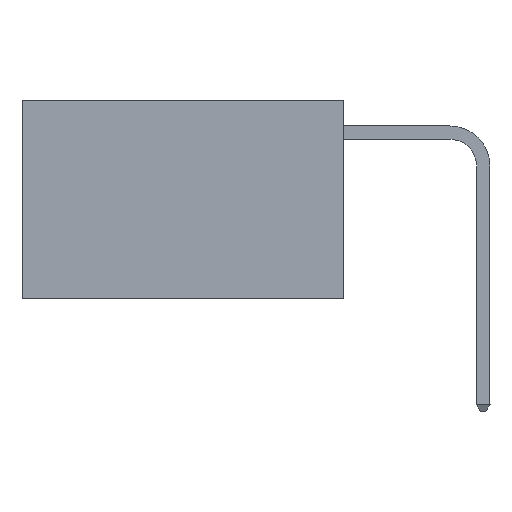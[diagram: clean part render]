
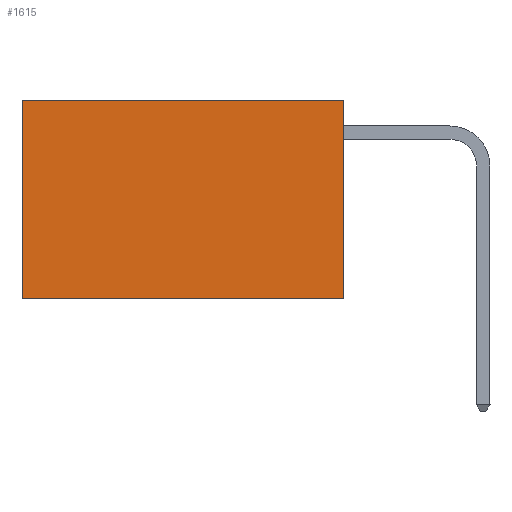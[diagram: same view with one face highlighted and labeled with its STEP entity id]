
A CAD part, left-side view. The second image highlights one B-rep face of the part: STEP entity #1615.
In plain terms, the highlighted planar face has unit normal (-1, 0, 0).
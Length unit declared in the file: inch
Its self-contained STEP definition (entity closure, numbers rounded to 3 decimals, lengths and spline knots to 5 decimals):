
#1 = LINE ( 'NONE', #4993, #1832 ) ;
#524 = CARTESIAN_POINT ( 'NONE',  ( 0.2625, 0., 0. ) ) ;
#731 = VERTEX_POINT ( 'NONE', #9139 ) ;
#1536 = CARTESIAN_POINT ( 'NONE',  ( 0.2625, 0.6, 0. ) ) ;
#1544 = VERTEX_POINT ( 'NONE', #2922 ) ;
#1615 = ADVANCED_FACE ( 'NONE', ( #4581 ), #5509, .F. ) ;
#1832 = VECTOR ( 'NONE', #2726, 39.37008 ) ;
#2323 = VECTOR ( 'NONE', #4527, 39.37008 ) ;
#2660 = DIRECTION ( 'NONE',  ( 1., 0., 0. ) ) ;
#2726 = DIRECTION ( 'NONE',  ( 0., 1., 0. ) ) ;
#2850 = VERTEX_POINT ( 'NONE', #5154 ) ;
#2922 = CARTESIAN_POINT ( 'NONE',  ( 0.2625, 0.6, 0. ) ) ;
#3022 = CARTESIAN_POINT ( 'NONE',  ( 0.2625, 0., 0. ) ) ;
#3250 = ORIENTED_EDGE ( 'NONE', *, *, #3322, .F. ) ;
#3322 = EDGE_CURVE ( 'NONE', #731, #2850, #1, .T. ) ;
#3621 = VECTOR ( 'NONE', #7573, 39.37008 ) ;
#3869 = LINE ( 'NONE', #3022, #3621 ) ;
#4019 = LINE ( 'NONE', #524, #7580 ) ;
#4245 = DIRECTION ( 'NONE',  ( 0., 0., -1. ) ) ;
#4527 = DIRECTION ( 'NONE',  ( 0., 0., -1. ) ) ;
#4581 = FACE_OUTER_BOUND ( 'NONE', #9106, .T. ) ;
#4606 = EDGE_CURVE ( 'NONE', #4980, #731, #4019, .T. ) ;
#4980 = VERTEX_POINT ( 'NONE', #7765 ) ;
#4993 = CARTESIAN_POINT ( 'NONE',  ( 0.2625, 0., -0.37 ) ) ;
#5154 = CARTESIAN_POINT ( 'NONE',  ( 0.2625, 0.6, -0.37 ) ) ;
#5509 = PLANE ( 'NONE',  #8423 ) ;
#6094 = LINE ( 'NONE', #1536, #2323 ) ;
#6120 = EDGE_CURVE ( 'NONE', #4980, #1544, #3869, .T. ) ;
#7141 = CARTESIAN_POINT ( 'NONE',  ( 0.2625, 0., 0. ) ) ;
#7573 = DIRECTION ( 'NONE',  ( 0., 1., 0. ) ) ;
#7580 = VECTOR ( 'NONE', #8839, 39.37008 ) ;
#7765 = CARTESIAN_POINT ( 'NONE',  ( 0.2625, 0., 0. ) ) ;
#8043 = EDGE_CURVE ( 'NONE', #1544, #2850, #6094, .T. ) ;
#8049 = ORIENTED_EDGE ( 'NONE', *, *, #6120, .T. ) ;
#8233 = ORIENTED_EDGE ( 'NONE', *, *, #8043, .T. ) ;
#8423 = AXIS2_PLACEMENT_3D ( 'NONE', #7141, #2660, #4245 ) ;
#8839 = DIRECTION ( 'NONE',  ( 0., 0., -1. ) ) ;
#9106 = EDGE_LOOP ( 'NONE', ( #8233, #3250, #9557, #8049 ) ) ;
#9139 = CARTESIAN_POINT ( 'NONE',  ( 0.2625, 0., -0.37 ) ) ;
#9557 = ORIENTED_EDGE ( 'NONE', *, *, #4606, .F. ) ;
